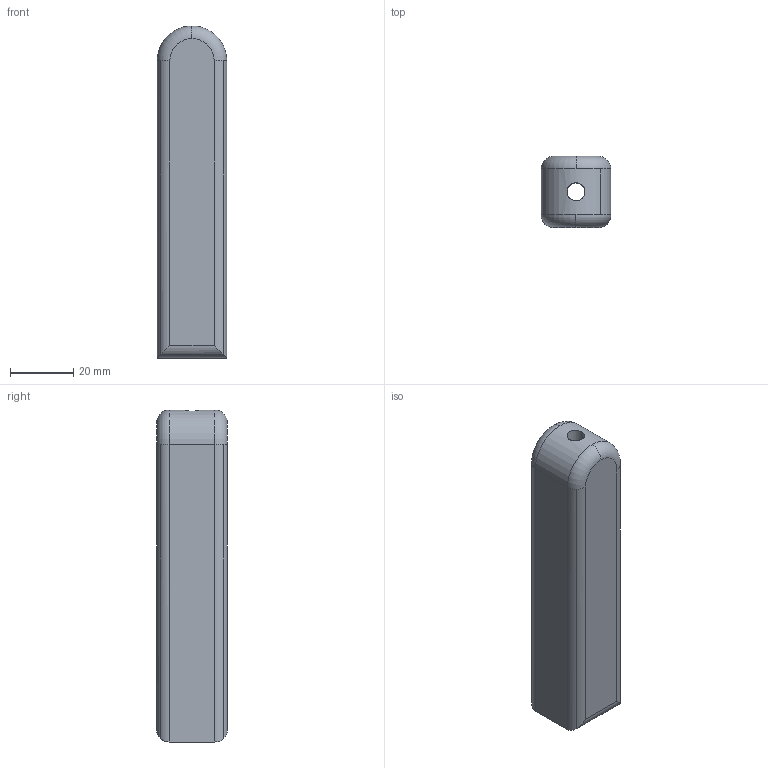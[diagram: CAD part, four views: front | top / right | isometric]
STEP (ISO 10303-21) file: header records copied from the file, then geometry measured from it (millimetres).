
FILE_DESCRIPTION(('STEP AP214'),'1');
FILE_NAME('barrel_scharf_smoothbore.stp','2019-06-25T13:25:05',(' '),(' '),'Spatial InterOp 3D',' ',' ');
FILE_SCHEMA(('AUTOMOTIVE_DESIGN { 1 0 10303 214 1 1 1 1 }'));
Length unit declared in the file: metre
Products named in the file (2): barrel_scharf_smoothbore; barrel_legal_verbessert
Assembly tree (1 placements, depth 2):
  barrel_scharf_smoothbore
    barrel_legal_verbessert
Bounding box: 22 x 22.4 x 104.9 mm (x, y, z)
Volume: 46239.2 mm3; surface area: 10948.6 mm2
Topology: 1 solids, 1 shells, 31 faces, 69 edges, 42 vertices
Faces by surface type: cylinder 20, plane 7, torus 4
Entity records: 1231 total; most frequent: CARTESIAN_POINT 210, DIRECTION 171, ORIENTED_EDGE 138, AXIS2_PLACEMENT_3D 71, EDGE_CURVE 69, VERTEX_POINT 42, EDGE_LOOP 35, STYLED_ITEM 32
